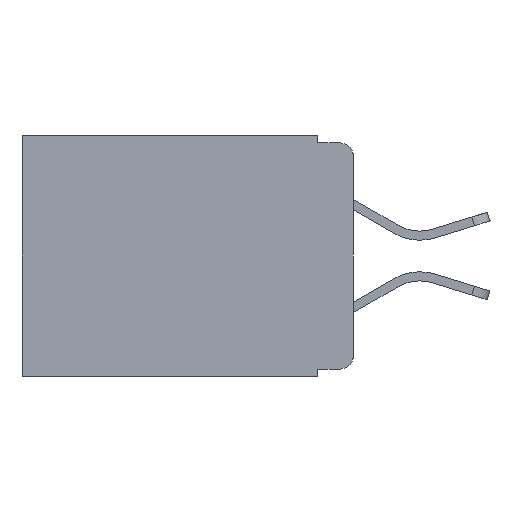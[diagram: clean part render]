
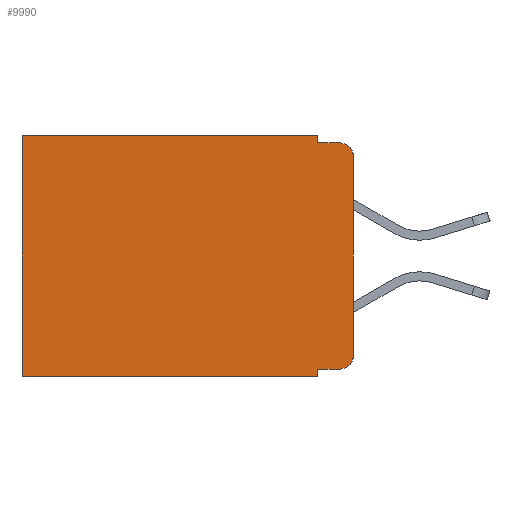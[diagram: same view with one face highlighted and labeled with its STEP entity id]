
A CAD part, left-side view. The second image highlights one B-rep face of the part: STEP entity #9990.
In plain terms, the highlighted planar face has unit normal (-1, 0, 0).
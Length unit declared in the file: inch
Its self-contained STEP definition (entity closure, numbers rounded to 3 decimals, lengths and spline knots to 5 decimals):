
#388 = DIRECTION ( 'NONE',  ( 0., 0., -1. ) ) ;
#398 = LINE ( 'NONE', #4478, #9776 ) ;
#488 = DIRECTION ( 'NONE',  ( 0., 0., -1. ) ) ;
#762 = EDGE_CURVE ( 'NONE', #4540, #11377, #1280, .T. ) ;
#765 = DIRECTION ( 'NONE',  ( 0., 1., 0. ) ) ;
#776 = DIRECTION ( 'NONE',  ( 0., 0., -1. ) ) ;
#1042 = LINE ( 'NONE', #4937, #1045 ) ;
#1045 = VECTOR ( 'NONE', #3757, 39.37008 ) ;
#1175 = AXIS2_PLACEMENT_3D ( 'NONE', #16782, #1746, #17974 ) ;
#1280 = LINE ( 'NONE', #4173, #15749 ) ;
#1282 = CARTESIAN_POINT ( 'NONE',  ( 0.298, 0.02, -0.01 ) ) ;
#1746 = DIRECTION ( 'NONE',  ( 1., 0., 0. ) ) ;
#2012 = CARTESIAN_POINT ( 'NONE',  ( 0.298, 0.473, -0.343 ) ) ;
#2808 = CARTESIAN_POINT ( 'NONE',  ( 0.298, 0.051, -0.333 ) ) ;
#3088 = ORIENTED_EDGE ( 'NONE', *, *, #9486, .T. ) ;
#3091 = EDGE_CURVE ( 'NONE', #13937, #11105, #1042, .T. ) ;
#3372 = CIRCLE ( 'NONE', #17948, 0.02 ) ;
#3476 = LINE ( 'NONE', #9009, #15920 ) ;
#3757 = DIRECTION ( 'NONE',  ( 0., -1., 0. ) ) ;
#3985 = LINE ( 'NONE', #13670, #14470 ) ;
#4173 = CARTESIAN_POINT ( 'NONE',  ( 0.298, 0., -0.343 ) ) ;
#4478 = CARTESIAN_POINT ( 'NONE',  ( 0.298, 0., 0. ) ) ;
#4540 = VERTEX_POINT ( 'NONE', #14254 ) ;
#4676 = DIRECTION ( 'NONE',  ( -1., 0., 0. ) ) ;
#4877 = LINE ( 'NONE', #14567, #12653 ) ;
#4937 = CARTESIAN_POINT ( 'NONE',  ( 0.298, 0.051, -0.01 ) ) ;
#5099 = CARTESIAN_POINT ( 'NONE',  ( 0.298, 0.051, 0. ) ) ;
#5102 = LINE ( 'NONE', #13242, #8056 ) ;
#5143 = CARTESIAN_POINT ( 'NONE',  ( 0.298, 0., -0.03 ) ) ;
#5355 = CIRCLE ( 'NONE', #15587, 0.02 ) ;
#5403 = DIRECTION ( 'NONE',  ( 0., 0., -1. ) ) ;
#5726 = PLANE ( 'NONE',  #1175 ) ;
#5933 = DIRECTION ( 'NONE',  ( 0., 0., -1. ) ) ;
#6078 = DIRECTION ( 'NONE',  ( 0., 0., -1. ) ) ;
#6179 = ORIENTED_EDGE ( 'NONE', *, *, #762, .F. ) ;
#6220 = CARTESIAN_POINT ( 'NONE',  ( 0.298, 0.02, -0.313 ) ) ;
#6770 = LINE ( 'NONE', #13818, #13225 ) ;
#7201 = DIRECTION ( 'NONE',  ( -1., 0., 0. ) ) ;
#7257 = FACE_OUTER_BOUND ( 'NONE', #17573, .T. ) ;
#7334 = EDGE_CURVE ( 'NONE', #17395, #17086, #5102, .T. ) ;
#7916 = CARTESIAN_POINT ( 'NONE',  ( 0.298, 0.02, -0.333 ) ) ;
#8056 = VECTOR ( 'NONE', #765, 39.37008 ) ;
#8078 = ORIENTED_EDGE ( 'NONE', *, *, #9719, .T. ) ;
#8448 = ORIENTED_EDGE ( 'NONE', *, *, #14080, .F. ) ;
#8816 = ORIENTED_EDGE ( 'NONE', *, *, #7334, .T. ) ;
#9009 = CARTESIAN_POINT ( 'NONE',  ( 0.298, 0.051, 0. ) ) ;
#9289 = VERTEX_POINT ( 'NONE', #7916 ) ;
#9447 = VERTEX_POINT ( 'NONE', #9743 ) ;
#9486 = EDGE_CURVE ( 'NONE', #16661, #11105, #5355, .T. ) ;
#9719 = EDGE_CURVE ( 'NONE', #16889, #9289, #3985, .T. ) ;
#9743 = CARTESIAN_POINT ( 'NONE',  ( 0.298, 0., -0.313 ) ) ;
#9776 = VECTOR ( 'NONE', #5933, 39.37008 ) ;
#9990 = ADVANCED_FACE ( 'NONE', ( #7257 ), #5726, .F. ) ;
#11105 = VERTEX_POINT ( 'NONE', #1282 ) ;
#11231 = CARTESIAN_POINT ( 'NONE',  ( 0.298, 0.051, -0.01 ) ) ;
#11265 = CARTESIAN_POINT ( 'NONE',  ( 0.298, 0.02, -0.03 ) ) ;
#11377 = VERTEX_POINT ( 'NONE', #2012 ) ;
#12103 = CARTESIAN_POINT ( 'NONE',  ( 0.298, 0.473, 0. ) ) ;
#12276 = ORIENTED_EDGE ( 'NONE', *, *, #17447, .T. ) ;
#12653 = VECTOR ( 'NONE', #6078, 39.37008 ) ;
#13225 = VECTOR ( 'NONE', #5403, 39.37008 ) ;
#13242 = CARTESIAN_POINT ( 'NONE',  ( 0.298, 0., 0. ) ) ;
#13670 = CARTESIAN_POINT ( 'NONE',  ( 0.298, 0.051, -0.333 ) ) ;
#13818 = CARTESIAN_POINT ( 'NONE',  ( 0.298, 0.473, 0. ) ) ;
#13937 = VERTEX_POINT ( 'NONE', #11231 ) ;
#14038 = DIRECTION ( 'NONE',  ( 0., 1., 0. ) ) ;
#14080 = EDGE_CURVE ( 'NONE', #16889, #4540, #4877, .T. ) ;
#14169 = EDGE_CURVE ( 'NONE', #17086, #11377, #6770, .T. ) ;
#14254 = CARTESIAN_POINT ( 'NONE',  ( 0.298, 0.051, -0.343 ) ) ;
#14470 = VECTOR ( 'NONE', #16325, 39.37008 ) ;
#14567 = CARTESIAN_POINT ( 'NONE',  ( 0.298, 0.051, 0. ) ) ;
#15453 = ORIENTED_EDGE ( 'NONE', *, *, #3091, .F. ) ;
#15587 = AXIS2_PLACEMENT_3D ( 'NONE', #11265, #7201, #388 ) ;
#15749 = VECTOR ( 'NONE', #14038, 39.37008 ) ;
#15920 = VECTOR ( 'NONE', #488, 39.37008 ) ;
#16325 = DIRECTION ( 'NONE',  ( 0., -1., 0. ) ) ;
#16661 = VERTEX_POINT ( 'NONE', #5143 ) ;
#16782 = CARTESIAN_POINT ( 'NONE',  ( 0.298, 0., 0. ) ) ;
#16877 = ORIENTED_EDGE ( 'NONE', *, *, #17847, .F. ) ;
#16889 = VERTEX_POINT ( 'NONE', #2808 ) ;
#17034 = ORIENTED_EDGE ( 'NONE', *, *, #18022, .F. ) ;
#17086 = VERTEX_POINT ( 'NONE', #12103 ) ;
#17137 = ORIENTED_EDGE ( 'NONE', *, *, #14169, .T. ) ;
#17395 = VERTEX_POINT ( 'NONE', #5099 ) ;
#17447 = EDGE_CURVE ( 'NONE', #9289, #9447, #3372, .T. ) ;
#17573 = EDGE_LOOP ( 'NONE', ( #16877, #3088, #15453, #17034, #8816, #17137, #6179, #8448, #8078, #12276 ) ) ;
#17847 = EDGE_CURVE ( 'NONE', #16661, #9447, #398, .T. ) ;
#17948 = AXIS2_PLACEMENT_3D ( 'NONE', #6220, #4676, #776 ) ;
#17974 = DIRECTION ( 'NONE',  ( 0., 0., -1. ) ) ;
#18022 = EDGE_CURVE ( 'NONE', #17395, #13937, #3476, .T. ) ;
